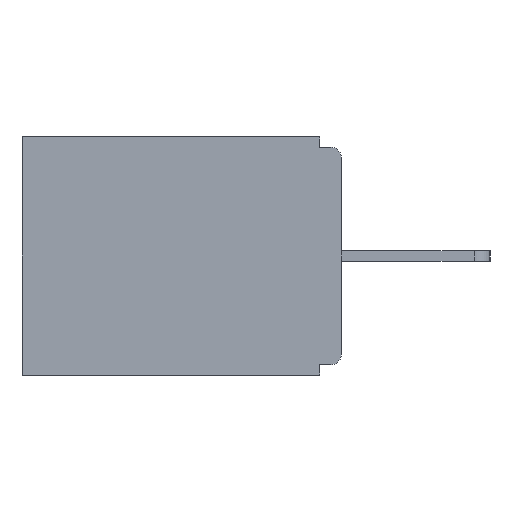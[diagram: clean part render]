
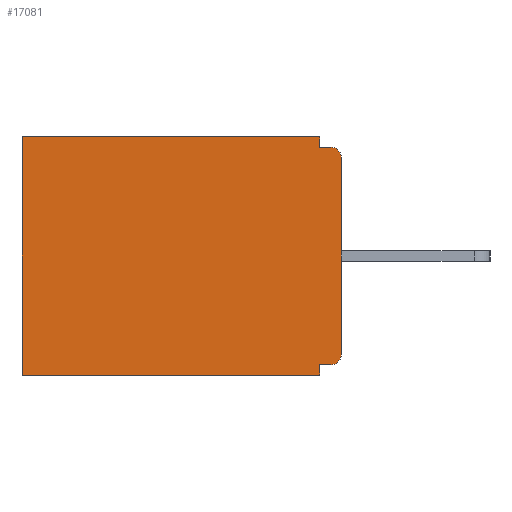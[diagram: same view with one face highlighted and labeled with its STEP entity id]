
A CAD part, left-side view. The second image highlights one B-rep face of the part: STEP entity #17081.
In plain terms, the highlighted planar face has unit normal (-1, 0, 0).
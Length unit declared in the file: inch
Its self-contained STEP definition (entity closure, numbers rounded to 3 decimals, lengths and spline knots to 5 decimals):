
#251 = CARTESIAN_POINT ( 'NONE',  ( 0.298, 0.015, -0.015 ) ) ;
#281 = VERTEX_POINT ( 'NONE', #21812 ) ;
#414 = LINE ( 'NONE', #9238, #1161 ) ;
#486 = CARTESIAN_POINT ( 'NONE',  ( 0.298, 0.031, -0.328 ) ) ;
#807 = CARTESIAN_POINT ( 'NONE',  ( 0.298, 0.015, -0.313 ) ) ;
#835 = CARTESIAN_POINT ( 'NONE',  ( 0.298, 0.015, -0.328 ) ) ;
#1063 = ORIENTED_EDGE ( 'NONE', *, *, #22555, .T. ) ;
#1084 = DIRECTION ( 'NONE',  ( 0., 0., -1. ) ) ;
#1161 = VECTOR ( 'NONE', #4076, 39.37008 ) ;
#1187 = ORIENTED_EDGE ( 'NONE', *, *, #9909, .T. ) ;
#1280 = DIRECTION ( 'NONE',  ( 0., 0., -1. ) ) ;
#1463 = EDGE_CURVE ( 'NONE', #281, #11215, #1865, .T. ) ;
#1592 = DIRECTION ( 'NONE',  ( 0., 0., -1. ) ) ;
#1865 = LINE ( 'NONE', #16433, #23186 ) ;
#2414 = CARTESIAN_POINT ( 'NONE',  ( 0.298, 0., -0.328 ) ) ;
#2532 = CARTESIAN_POINT ( 'NONE',  ( 0.298, 0.46, 0. ) ) ;
#2657 = PLANE ( 'NONE',  #23175 ) ;
#3071 = VERTEX_POINT ( 'NONE', #6766 ) ;
#3269 = CARTESIAN_POINT ( 'NONE',  ( 0.298, 0.031, -0.343 ) ) ;
#4076 = DIRECTION ( 'NONE',  ( 0., 1., 0. ) ) ;
#4093 = VECTOR ( 'NONE', #1592, 39.37008 ) ;
#4189 = FACE_OUTER_BOUND ( 'NONE', #13971, .T. ) ;
#4525 = DIRECTION ( 'NONE',  ( 1., 0., 0. ) ) ;
#4598 = DIRECTION ( 'NONE',  ( -1., 0., 0. ) ) ;
#4708 = LINE ( 'NONE', #9976, #14404 ) ;
#4798 = EDGE_CURVE ( 'NONE', #11215, #23449, #4708, .T. ) ;
#5060 = VECTOR ( 'NONE', #7818, 39.37008 ) ;
#6766 = CARTESIAN_POINT ( 'NONE',  ( 0.298, 0.031, -0.343 ) ) ;
#7388 = VERTEX_POINT ( 'NONE', #11928 ) ;
#7417 = ORIENTED_EDGE ( 'NONE', *, *, #9080, .F. ) ;
#7818 = DIRECTION ( 'NONE',  ( 0., 1., 0. ) ) ;
#7828 = DIRECTION ( 'NONE',  ( 0., 0., -1. ) ) ;
#8171 = VERTEX_POINT ( 'NONE', #8610 ) ;
#8414 = ORIENTED_EDGE ( 'NONE', *, *, #16851, .F. ) ;
#8460 = ORIENTED_EDGE ( 'NONE', *, *, #11792, .T. ) ;
#8576 = EDGE_CURVE ( 'NONE', #11328, #22242, #18651, .T. ) ;
#8610 = CARTESIAN_POINT ( 'NONE',  ( 0.298, 0.46, -0.343 ) ) ;
#9080 = EDGE_CURVE ( 'NONE', #7388, #18106, #21223, .T. ) ;
#9174 = AXIS2_PLACEMENT_3D ( 'NONE', #19226, #17434, #1084 ) ;
#9238 = CARTESIAN_POINT ( 'NONE',  ( 0.298, 0., -0.343 ) ) ;
#9508 = VECTOR ( 'NONE', #1280, 39.37008 ) ;
#9747 = EDGE_CURVE ( 'NONE', #11251, #8171, #20438, .T. ) ;
#9909 = EDGE_CURVE ( 'NONE', #7388, #23449, #15277, .T. ) ;
#9976 = CARTESIAN_POINT ( 'NONE',  ( 0.298, 0., -0.015 ) ) ;
#10339 = DIRECTION ( 'NONE',  ( 0., 0., -1. ) ) ;
#11215 = VERTEX_POINT ( 'NONE', #14924 ) ;
#11251 = VERTEX_POINT ( 'NONE', #20305 ) ;
#11328 = VERTEX_POINT ( 'NONE', #835 ) ;
#11356 = ORIENTED_EDGE ( 'NONE', *, *, #8576, .F. ) ;
#11690 = DIRECTION ( 'NONE',  ( 0., 0., -1. ) ) ;
#11777 = CARTESIAN_POINT ( 'NONE',  ( 0.298, 0., 0. ) ) ;
#11792 = EDGE_CURVE ( 'NONE', #11328, #18106, #18230, .T. ) ;
#11928 = CARTESIAN_POINT ( 'NONE',  ( 0.298, 0., -0.03 ) ) ;
#11996 = DIRECTION ( 'NONE',  ( 0., -1., 0. ) ) ;
#12107 = AXIS2_PLACEMENT_3D ( 'NONE', #807, #4598, #10339 ) ;
#12331 = ORIENTED_EDGE ( 'NONE', *, *, #1463, .F. ) ;
#12704 = CARTESIAN_POINT ( 'NONE',  ( 0.298, 0., 0. ) ) ;
#13971 = EDGE_LOOP ( 'NONE', ( #1187, #22563, #12331, #1063, #19624, #21195, #8414, #11356, #8460, #7417 ) ) ;
#14404 = VECTOR ( 'NONE', #11996, 39.37008 ) ;
#14924 = CARTESIAN_POINT ( 'NONE',  ( 0.298, 0.031, -0.015 ) ) ;
#14963 = CARTESIAN_POINT ( 'NONE',  ( 0.298, 0., -0.313 ) ) ;
#15259 = VECTOR ( 'NONE', #11690, 39.37008 ) ;
#15277 = CIRCLE ( 'NONE', #9174, 0.015 ) ;
#16433 = CARTESIAN_POINT ( 'NONE',  ( 0.298, 0.031, -0.343 ) ) ;
#16851 = EDGE_CURVE ( 'NONE', #22242, #3071, #23323, .T. ) ;
#16857 = DIRECTION ( 'NONE',  ( 0., 1., 0. ) ) ;
#17081 = ADVANCED_FACE ( 'NONE', ( #4189 ), #2657, .F. ) ;
#17434 = DIRECTION ( 'NONE',  ( -1., 0., 0. ) ) ;
#17885 = VECTOR ( 'NONE', #16857, 39.37008 ) ;
#18103 = EDGE_CURVE ( 'NONE', #3071, #8171, #414, .T. ) ;
#18106 = VERTEX_POINT ( 'NONE', #14963 ) ;
#18230 = CIRCLE ( 'NONE', #12107, 0.015 ) ;
#18651 = LINE ( 'NONE', #2414, #17885 ) ;
#18778 = CARTESIAN_POINT ( 'NONE',  ( 0.298, 0., 0. ) ) ;
#19226 = CARTESIAN_POINT ( 'NONE',  ( 0.298, 0.015, -0.03 ) ) ;
#19624 = ORIENTED_EDGE ( 'NONE', *, *, #9747, .T. ) ;
#20305 = CARTESIAN_POINT ( 'NONE',  ( 0.298, 0.46, 0. ) ) ;
#20438 = LINE ( 'NONE', #2532, #15259 ) ;
#21195 = ORIENTED_EDGE ( 'NONE', *, *, #18103, .F. ) ;
#21223 = LINE ( 'NONE', #11777, #9508 ) ;
#21812 = CARTESIAN_POINT ( 'NONE',  ( 0.298, 0.031, 0. ) ) ;
#22030 = LINE ( 'NONE', #12704, #5060 ) ;
#22242 = VERTEX_POINT ( 'NONE', #486 ) ;
#22555 = EDGE_CURVE ( 'NONE', #281, #11251, #22030, .T. ) ;
#22563 = ORIENTED_EDGE ( 'NONE', *, *, #4798, .F. ) ;
#22694 = DIRECTION ( 'NONE',  ( 0., 0., -1. ) ) ;
#23175 = AXIS2_PLACEMENT_3D ( 'NONE', #18778, #4525, #22694 ) ;
#23186 = VECTOR ( 'NONE', #7828, 39.37008 ) ;
#23323 = LINE ( 'NONE', #3269, #4093 ) ;
#23449 = VERTEX_POINT ( 'NONE', #251 ) ;
